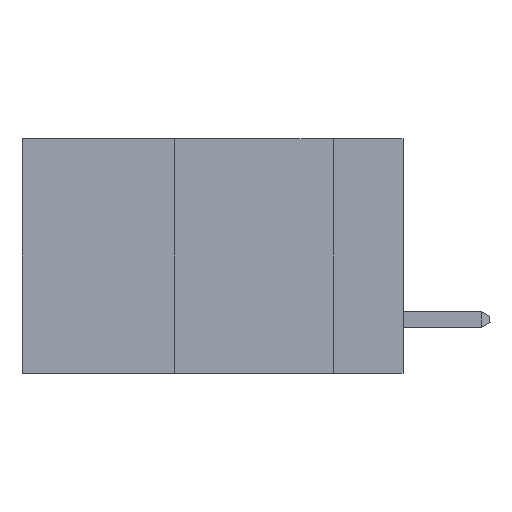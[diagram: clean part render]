
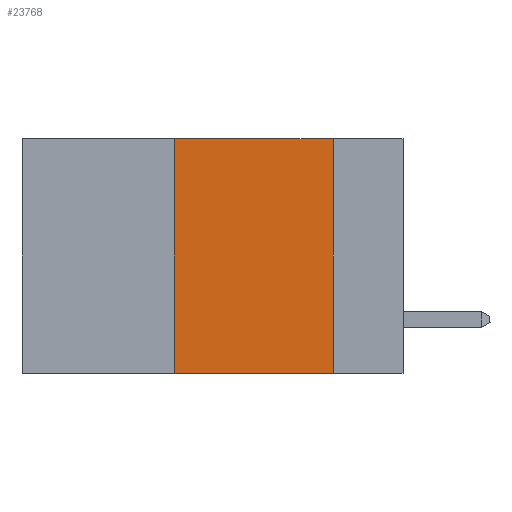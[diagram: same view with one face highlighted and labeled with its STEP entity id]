
A CAD part, left-side view. The second image highlights one B-rep face of the part: STEP entity #23768.
In plain terms, the highlighted planar face has unit normal (-1, 0, 0).
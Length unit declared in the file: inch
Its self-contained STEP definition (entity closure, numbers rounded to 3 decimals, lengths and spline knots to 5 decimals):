
#366 = CARTESIAN_POINT ( 'NONE',  ( 0., 0.36, -0.37 ) ) ;
#2818 = CARTESIAN_POINT ( 'NONE',  ( 0., 0.36, 0. ) ) ;
#3642 = EDGE_CURVE ( 'NONE', #22081, #6889, #29139, .T. ) ;
#3695 = VECTOR ( 'NONE', #8775, 39.37008 ) ;
#6449 = CARTESIAN_POINT ( 'NONE',  ( 0., 0.11, 0. ) ) ;
#6645 = CARTESIAN_POINT ( 'NONE',  ( 0., 0.11, 0. ) ) ;
#6889 = VERTEX_POINT ( 'NONE', #8320 ) ;
#7519 = DIRECTION ( 'NONE',  ( 0., 0., -1. ) ) ;
#8320 = CARTESIAN_POINT ( 'NONE',  ( 0., 0.11, -0.37 ) ) ;
#8589 = EDGE_CURVE ( 'NONE', #33650, #22081, #36150, .T. ) ;
#8775 = DIRECTION ( 'NONE',  ( 0., 0., 1. ) ) ;
#11489 = PLANE ( 'NONE',  #38539 ) ;
#11676 = FACE_OUTER_BOUND ( 'NONE', #39375, .T. ) ;
#13036 = LINE ( 'NONE', #15817, #3695 ) ;
#13438 = DIRECTION ( 'NONE',  ( 0., 0., -1. ) ) ;
#14557 = DIRECTION ( 'NONE',  ( 0., -1., 0. ) ) ;
#15817 = CARTESIAN_POINT ( 'NONE',  ( 0., 0.36, 0. ) ) ;
#18220 = CARTESIAN_POINT ( 'NONE',  ( 0., 0.6, -0.37 ) ) ;
#19407 = ORIENTED_EDGE ( 'NONE', *, *, #34723, .F. ) ;
#20424 = EDGE_CURVE ( 'NONE', #24687, #6889, #26197, .T. ) ;
#20830 = VECTOR ( 'NONE', #43824, 39.37008 ) ;
#22081 = VERTEX_POINT ( 'NONE', #6449 ) ;
#22552 = CARTESIAN_POINT ( 'NONE',  ( 0., 0.6, 0. ) ) ;
#23516 = VECTOR ( 'NONE', #14557, 39.37008 ) ;
#23768 = ADVANCED_FACE ( 'NONE', ( #11676 ), #11489, .F. ) ;
#24687 = VERTEX_POINT ( 'NONE', #366 ) ;
#25286 = ORIENTED_EDGE ( 'NONE', *, *, #20424, .T. ) ;
#26197 = LINE ( 'NONE', #18220, #23516 ) ;
#29139 = LINE ( 'NONE', #6645, #30827 ) ;
#30827 = VECTOR ( 'NONE', #13438, 39.37008 ) ;
#31446 = ORIENTED_EDGE ( 'NONE', *, *, #3642, .F. ) ;
#33650 = VERTEX_POINT ( 'NONE', #2818 ) ;
#34723 = EDGE_CURVE ( 'NONE', #24687, #33650, #13036, .T. ) ;
#35569 = CARTESIAN_POINT ( 'NONE',  ( 0., 0.6, 0. ) ) ;
#35868 = DIRECTION ( 'NONE',  ( 1., 0., 0. ) ) ;
#36150 = LINE ( 'NONE', #22552, #20830 ) ;
#38539 = AXIS2_PLACEMENT_3D ( 'NONE', #35569, #35868, #7519 ) ;
#39375 = EDGE_LOOP ( 'NONE', ( #31446, #42587, #19407, #25286 ) ) ;
#42587 = ORIENTED_EDGE ( 'NONE', *, *, #8589, .F. ) ;
#43824 = DIRECTION ( 'NONE',  ( 0., -1., 0. ) ) ;
